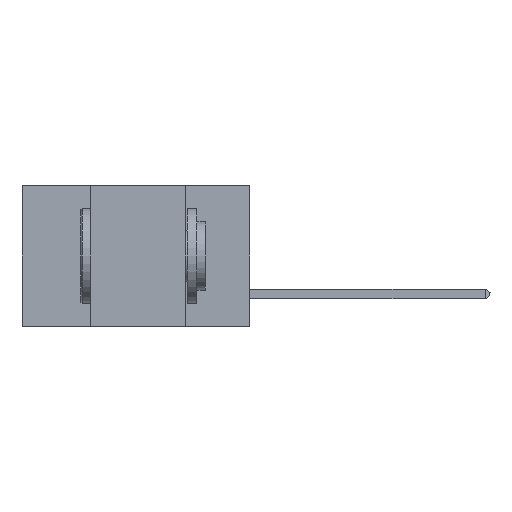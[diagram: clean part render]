
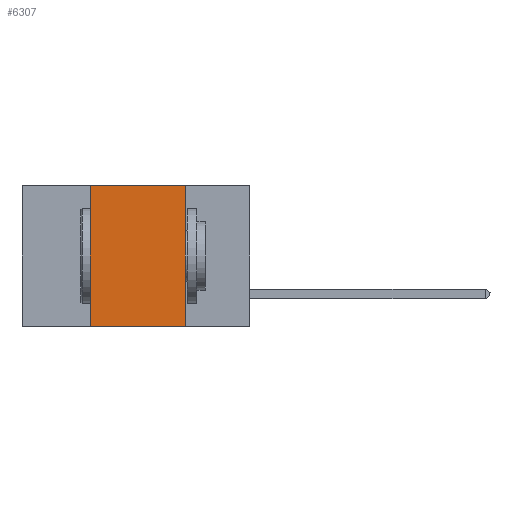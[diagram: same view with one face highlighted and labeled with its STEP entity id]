
A CAD part, left-side view. The second image highlights one B-rep face of the part: STEP entity #6307.
In plain terms, the highlighted planar face has unit normal (-1, 0, 0).
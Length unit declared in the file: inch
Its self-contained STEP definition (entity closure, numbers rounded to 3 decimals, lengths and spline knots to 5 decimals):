
#2437 = ORIENTED_EDGE ( 'NONE', *, *, #23467, .F. ) ;
#2702 = LINE ( 'NONE', #38648, #31617 ) ;
#5144 = DIRECTION ( 'NONE',  ( 0., -1., 0. ) ) ;
#6206 = CARTESIAN_POINT ( 'NONE',  ( 0., 0.17, 0. ) ) ;
#6307 = ADVANCED_FACE ( 'NONE', ( #12506 ), #23666, .F. ) ;
#7118 = CARTESIAN_POINT ( 'NONE',  ( 0., 0.17, -0.37 ) ) ;
#7229 = EDGE_CURVE ( 'NONE', #9589, #27721, #16271, .T. ) ;
#8317 = DIRECTION ( 'NONE',  ( 0., 0., -1. ) ) ;
#9561 = EDGE_LOOP ( 'NONE', ( #34561, #28104, #2437, #21254 ) ) ;
#9589 = VERTEX_POINT ( 'NONE', #6206 ) ;
#9846 = CARTESIAN_POINT ( 'NONE',  ( 0., 0.6, 0. ) ) ;
#11005 = CARTESIAN_POINT ( 'NONE',  ( 0., 0.42, 0. ) ) ;
#12506 = FACE_OUTER_BOUND ( 'NONE', #9561, .T. ) ;
#14238 = VECTOR ( 'NONE', #5144, 39.37008 ) ;
#15160 = DIRECTION ( 'NONE',  ( 0., 0., -1. ) ) ;
#15283 = VECTOR ( 'NONE', #15160, 39.37008 ) ;
#15706 = CARTESIAN_POINT ( 'NONE',  ( 0., 0.17, 0. ) ) ;
#16271 = LINE ( 'NONE', #15706, #15283 ) ;
#17583 = DIRECTION ( 'NONE',  ( 0., -1., 0. ) ) ;
#17628 = VERTEX_POINT ( 'NONE', #24939 ) ;
#20914 = EDGE_CURVE ( 'NONE', #36931, #9589, #24678, .T. ) ;
#21254 = ORIENTED_EDGE ( 'NONE', *, *, #34884, .T. ) ;
#23467 = EDGE_CURVE ( 'NONE', #17628, #36931, #36339, .T. ) ;
#23666 = PLANE ( 'NONE',  #36812 ) ;
#24678 = LINE ( 'NONE', #9846, #14238 ) ;
#24939 = CARTESIAN_POINT ( 'NONE',  ( 0., 0.42, -0.37 ) ) ;
#27721 = VERTEX_POINT ( 'NONE', #7118 ) ;
#28104 = ORIENTED_EDGE ( 'NONE', *, *, #20914, .F. ) ;
#29711 = VECTOR ( 'NONE', #38358, 39.37008 ) ;
#31617 = VECTOR ( 'NONE', #17583, 39.37008 ) ;
#32656 = DIRECTION ( 'NONE',  ( 1., 0., 0. ) ) ;
#32915 = CARTESIAN_POINT ( 'NONE',  ( 0., 0.6, 0. ) ) ;
#32967 = CARTESIAN_POINT ( 'NONE',  ( 0., 0.42, 0. ) ) ;
#34561 = ORIENTED_EDGE ( 'NONE', *, *, #7229, .F. ) ;
#34884 = EDGE_CURVE ( 'NONE', #17628, #27721, #2702, .T. ) ;
#36339 = LINE ( 'NONE', #11005, #29711 ) ;
#36812 = AXIS2_PLACEMENT_3D ( 'NONE', #32915, #32656, #8317 ) ;
#36931 = VERTEX_POINT ( 'NONE', #32967 ) ;
#38358 = DIRECTION ( 'NONE',  ( 0., 0., 1. ) ) ;
#38648 = CARTESIAN_POINT ( 'NONE',  ( 0., 0.6, -0.37 ) ) ;
